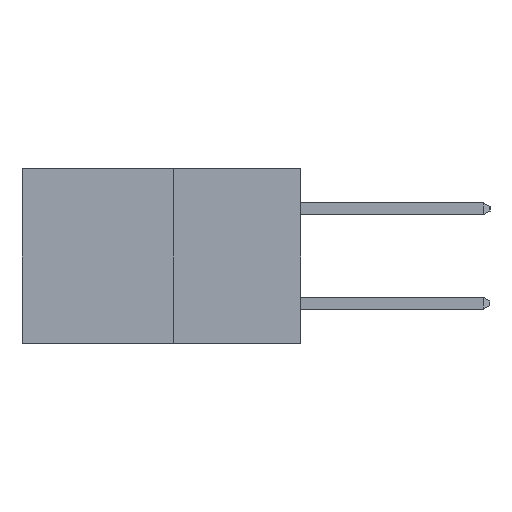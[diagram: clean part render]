
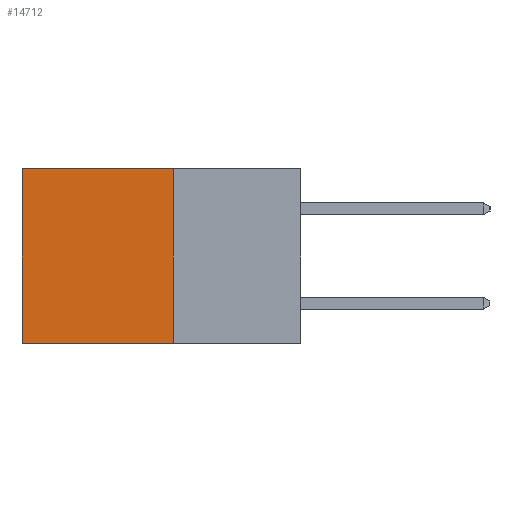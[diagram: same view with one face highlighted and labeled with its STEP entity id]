
A CAD part, left-side view. The second image highlights one B-rep face of the part: STEP entity #14712.
In plain terms, the highlighted planar face has unit normal (-1, 0, 0).
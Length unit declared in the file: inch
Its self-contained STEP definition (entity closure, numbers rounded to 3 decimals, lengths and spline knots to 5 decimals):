
#87 = ORIENTED_EDGE ( 'NONE', *, *, #21927, .T. ) ;
#846 = DIRECTION ( 'NONE',  ( 0., 1., 0. ) ) ;
#1895 = CARTESIAN_POINT ( 'NONE',  ( 0.277, 0.59, -0.37 ) ) ;
#3443 = VERTEX_POINT ( 'NONE', #18987 ) ;
#3782 = LINE ( 'NONE', #1895, #14002 ) ;
#5492 = PLANE ( 'NONE',  #11953 ) ;
#6334 = ORIENTED_EDGE ( 'NONE', *, *, #18121, .T. ) ;
#6672 = CARTESIAN_POINT ( 'NONE',  ( 0.277, 0.27, -0.37 ) ) ;
#8772 = CARTESIAN_POINT ( 'NONE',  ( 0.277, 0.27, 0. ) ) ;
#9400 = DIRECTION ( 'NONE',  ( 1., 0., 0. ) ) ;
#9708 = LINE ( 'NONE', #8772, #18523 ) ;
#9740 = VERTEX_POINT ( 'NONE', #21378 ) ;
#10273 = EDGE_CURVE ( 'NONE', #9740, #20434, #19007, .T. ) ;
#10679 = EDGE_LOOP ( 'NONE', ( #6334, #23911, #14647, #87 ) ) ;
#11627 = CARTESIAN_POINT ( 'NONE',  ( 0.277, 0.27, -0.37 ) ) ;
#11953 = AXIS2_PLACEMENT_3D ( 'NONE', #20613, #9400, #22484 ) ;
#12103 = FACE_OUTER_BOUND ( 'NONE', #10679, .T. ) ;
#13446 = DIRECTION ( 'NONE',  ( 0., 0., -1. ) ) ;
#13524 = DIRECTION ( 'NONE',  ( 0., 0., -1. ) ) ;
#14002 = VECTOR ( 'NONE', #13446, 39.37008 ) ;
#14647 = ORIENTED_EDGE ( 'NONE', *, *, #10273, .F. ) ;
#14712 = ADVANCED_FACE ( 'NONE', ( #12103 ), #5492, .F. ) ;
#15873 = VECTOR ( 'NONE', #846, 39.37008 ) ;
#16303 = DIRECTION ( 'NONE',  ( 0., 1., 0. ) ) ;
#18121 = EDGE_CURVE ( 'NONE', #20139, #3443, #3782, .T. ) ;
#18410 = VECTOR ( 'NONE', #13524, 39.37008 ) ;
#18523 = VECTOR ( 'NONE', #16303, 39.37008 ) ;
#18987 = CARTESIAN_POINT ( 'NONE',  ( 0.277, 0.59, -0.37 ) ) ;
#19007 = LINE ( 'NONE', #11627, #18410 ) ;
#20139 = VERTEX_POINT ( 'NONE', #24067 ) ;
#20434 = VERTEX_POINT ( 'NONE', #23081 ) ;
#20613 = CARTESIAN_POINT ( 'NONE',  ( 0.277, 0.27, -0.37 ) ) ;
#21377 = LINE ( 'NONE', #6672, #15873 ) ;
#21378 = CARTESIAN_POINT ( 'NONE',  ( 0.277, 0.27, 0. ) ) ;
#21927 = EDGE_CURVE ( 'NONE', #9740, #20139, #9708, .T. ) ;
#22257 = EDGE_CURVE ( 'NONE', #20434, #3443, #21377, .T. ) ;
#22484 = DIRECTION ( 'NONE',  ( 0., 0., -1. ) ) ;
#23081 = CARTESIAN_POINT ( 'NONE',  ( 0.277, 0.27, -0.37 ) ) ;
#23911 = ORIENTED_EDGE ( 'NONE', *, *, #22257, .F. ) ;
#24067 = CARTESIAN_POINT ( 'NONE',  ( 0.277, 0.59, 0. ) ) ;
